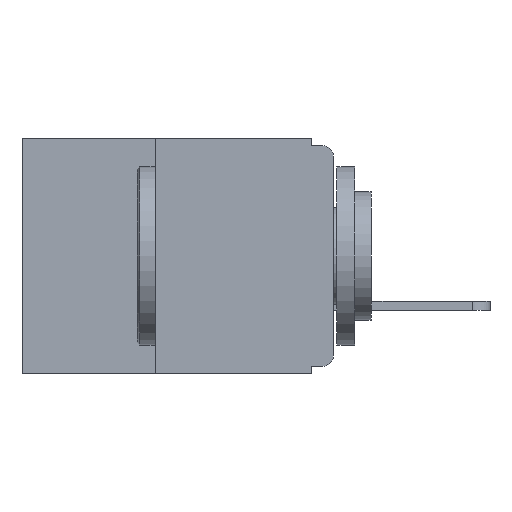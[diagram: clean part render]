
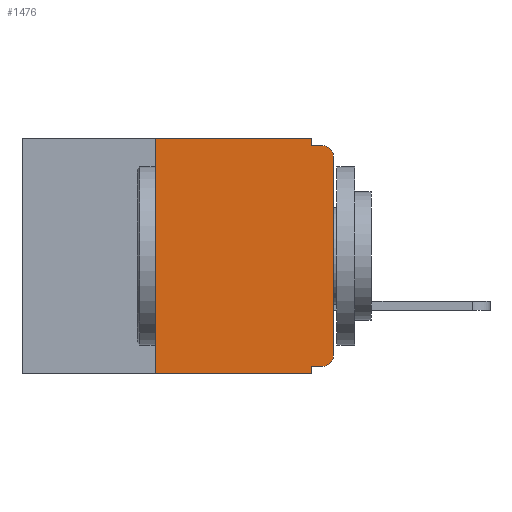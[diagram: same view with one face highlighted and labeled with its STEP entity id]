
A CAD part, left-side view. The second image highlights one B-rep face of the part: STEP entity #1476.
In plain terms, the highlighted planar face has unit normal (-1, 0, 0).
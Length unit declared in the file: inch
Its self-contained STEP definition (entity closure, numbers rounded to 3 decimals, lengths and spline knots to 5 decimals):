
#111 = AXIS2_PLACEMENT_3D ( 'NONE', #7053, #11717, #11775 ) ;
#161 = LINE ( 'NONE', #13754, #1239 ) ;
#196 = CARTESIAN_POINT ( 'NONE',  ( 0., 0.25, 0. ) ) ;
#199 = CARTESIAN_POINT ( 'NONE',  ( 0., 0.015, -0.32 ) ) ;
#306 = VECTOR ( 'NONE', #9654, 39.37008 ) ;
#314 = EDGE_CURVE ( 'NONE', #3916, #9724, #161, .T. ) ;
#711 = CARTESIAN_POINT ( 'NONE',  ( 0., 0.437, 0. ) ) ;
#770 = CARTESIAN_POINT ( 'NONE',  ( 0., 0., -0.305 ) ) ;
#943 = DIRECTION ( 'NONE',  ( 0., 0., -1. ) ) ;
#1239 = VECTOR ( 'NONE', #943, 39.37008 ) ;
#1400 = VERTEX_POINT ( 'NONE', #196 ) ;
#1412 = DIRECTION ( 'NONE',  ( 0., -1., 0. ) ) ;
#1476 = ADVANCED_FACE ( 'NONE', ( #4818 ), #5013, .F. ) ;
#1924 = ORIENTED_EDGE ( 'NONE', *, *, #6826, .T. ) ;
#2021 = EDGE_CURVE ( 'NONE', #9121, #7323, #12773, .T. ) ;
#2070 = CARTESIAN_POINT ( 'NONE',  ( 0., 0.015, -0.305 ) ) ;
#2258 = ORIENTED_EDGE ( 'NONE', *, *, #7403, .F. ) ;
#2858 = AXIS2_PLACEMENT_3D ( 'NONE', #6200, #2892, #9788 ) ;
#2892 = DIRECTION ( 'NONE',  ( 1., 0., 0. ) ) ;
#2958 = LINE ( 'NONE', #5090, #7041 ) ;
#3267 = CARTESIAN_POINT ( 'NONE',  ( 0., 0.031, -0.33 ) ) ;
#3762 = DIRECTION ( 'NONE',  ( 0., 1., 0. ) ) ;
#3875 = CARTESIAN_POINT ( 'NONE',  ( 0., 0.437, -0.33 ) ) ;
#3916 = VERTEX_POINT ( 'NONE', #4097 ) ;
#3945 = EDGE_CURVE ( 'NONE', #1400, #3916, #13807, .T. ) ;
#3999 = CARTESIAN_POINT ( 'NONE',  ( 0., 0.25, -0.33 ) ) ;
#4097 = CARTESIAN_POINT ( 'NONE',  ( 0., 0.031, 0. ) ) ;
#4326 = ORIENTED_EDGE ( 'NONE', *, *, #6544, .F. ) ;
#4818 = FACE_OUTER_BOUND ( 'NONE', #12631, .T. ) ;
#4906 = VECTOR ( 'NONE', #8888, 39.37008 ) ;
#5013 = PLANE ( 'NONE',  #2858 ) ;
#5090 = CARTESIAN_POINT ( 'NONE',  ( 0., 0., -0.01 ) ) ;
#5427 = DIRECTION ( 'NONE',  ( 0., -1., 0. ) ) ;
#5455 = LINE ( 'NONE', #6409, #7072 ) ;
#5850 = LINE ( 'NONE', #12915, #306 ) ;
#5953 = LINE ( 'NONE', #14316, #6135 ) ;
#6135 = VECTOR ( 'NONE', #3762, 39.37008 ) ;
#6200 = CARTESIAN_POINT ( 'NONE',  ( 0., 0.437, 0. ) ) ;
#6283 = AXIS2_PLACEMENT_3D ( 'NONE', #2070, #7737, #11314 ) ;
#6409 = CARTESIAN_POINT ( 'NONE',  ( 0., 0.25, -0.33 ) ) ;
#6419 = EDGE_CURVE ( 'NONE', #10501, #12755, #8917, .T. ) ;
#6544 = EDGE_CURVE ( 'NONE', #10501, #1400, #5455, .T. ) ;
#6826 = EDGE_CURVE ( 'NONE', #11536, #11667, #14383, .T. ) ;
#6869 = VERTEX_POINT ( 'NONE', #11844 ) ;
#7041 = VECTOR ( 'NONE', #7393, 39.37008 ) ;
#7053 = CARTESIAN_POINT ( 'NONE',  ( 0., 0.015, -0.025 ) ) ;
#7072 = VECTOR ( 'NONE', #14584, 39.37008 ) ;
#7213 = CARTESIAN_POINT ( 'NONE',  ( 0., 0.015, -0.01 ) ) ;
#7225 = EDGE_CURVE ( 'NONE', #9724, #11667, #2958, .T. ) ;
#7323 = VERTEX_POINT ( 'NONE', #770 ) ;
#7393 = DIRECTION ( 'NONE',  ( 0., -1., 0. ) ) ;
#7403 = EDGE_CURVE ( 'NONE', #6869, #12755, #10717, .T. ) ;
#7584 = EDGE_CURVE ( 'NONE', #9121, #6869, #5953, .T. ) ;
#7598 = CARTESIAN_POINT ( 'NONE',  ( 0., 0.031, -0.33 ) ) ;
#7737 = DIRECTION ( 'NONE',  ( -1., 0., 0. ) ) ;
#7970 = ORIENTED_EDGE ( 'NONE', *, *, #11053, .T. ) ;
#8032 = ORIENTED_EDGE ( 'NONE', *, *, #314, .F. ) ;
#8035 = CARTESIAN_POINT ( 'NONE',  ( 0., 0., -0.025 ) ) ;
#8170 = VECTOR ( 'NONE', #1412, 39.37008 ) ;
#8888 = DIRECTION ( 'NONE',  ( 0., 0., -1. ) ) ;
#8917 = LINE ( 'NONE', #3875, #8170 ) ;
#9060 = VECTOR ( 'NONE', #5427, 39.37008 ) ;
#9121 = VERTEX_POINT ( 'NONE', #199 ) ;
#9654 = DIRECTION ( 'NONE',  ( 0., 0., 1. ) ) ;
#9724 = VERTEX_POINT ( 'NONE', #14136 ) ;
#9788 = DIRECTION ( 'NONE',  ( 0., 0., -1. ) ) ;
#10501 = VERTEX_POINT ( 'NONE', #3999 ) ;
#10717 = LINE ( 'NONE', #7598, #4906 ) ;
#11053 = EDGE_CURVE ( 'NONE', #7323, #11536, #5850, .T. ) ;
#11314 = DIRECTION ( 'NONE',  ( 0., 0., -1. ) ) ;
#11536 = VERTEX_POINT ( 'NONE', #8035 ) ;
#11621 = ORIENTED_EDGE ( 'NONE', *, *, #7225, .F. ) ;
#11667 = VERTEX_POINT ( 'NONE', #7213 ) ;
#11717 = DIRECTION ( 'NONE',  ( -1., 0., 0. ) ) ;
#11775 = DIRECTION ( 'NONE',  ( 0., 0., -1. ) ) ;
#11844 = CARTESIAN_POINT ( 'NONE',  ( 0., 0.031, -0.32 ) ) ;
#12289 = ORIENTED_EDGE ( 'NONE', *, *, #7584, .F. ) ;
#12631 = EDGE_LOOP ( 'NONE', ( #7970, #1924, #11621, #8032, #14597, #4326, #13389, #2258, #12289, #13469 ) ) ;
#12755 = VERTEX_POINT ( 'NONE', #3267 ) ;
#12773 = CIRCLE ( 'NONE', #6283, 0.015 ) ;
#12915 = CARTESIAN_POINT ( 'NONE',  ( 0., 0., 0. ) ) ;
#13389 = ORIENTED_EDGE ( 'NONE', *, *, #6419, .T. ) ;
#13469 = ORIENTED_EDGE ( 'NONE', *, *, #2021, .T. ) ;
#13754 = CARTESIAN_POINT ( 'NONE',  ( 0., 0.031, 0. ) ) ;
#13807 = LINE ( 'NONE', #711, #9060 ) ;
#14136 = CARTESIAN_POINT ( 'NONE',  ( 0., 0.031, -0.01 ) ) ;
#14316 = CARTESIAN_POINT ( 'NONE',  ( 0., 0., -0.32 ) ) ;
#14383 = CIRCLE ( 'NONE', #111, 0.015 ) ;
#14584 = DIRECTION ( 'NONE',  ( 0., 0., 1. ) ) ;
#14597 = ORIENTED_EDGE ( 'NONE', *, *, #3945, .F. ) ;
